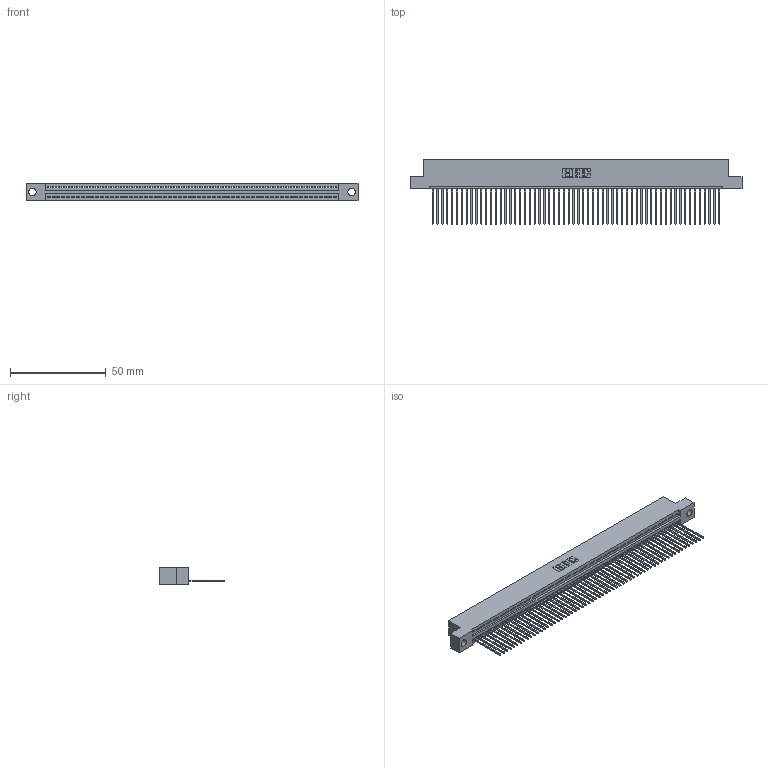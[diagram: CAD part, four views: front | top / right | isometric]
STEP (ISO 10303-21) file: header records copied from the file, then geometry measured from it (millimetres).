
FILE_DESCRIPTION (( 'STEP AP203' ), '1' );
FILE_NAME ('395-060-541-104.STEP', '2021-05-31T21:48:45', ( '' ), ( '' ), 'SwSTEP 2.0', 'SolidWorks 2020', '' );
FILE_SCHEMA (( 'CONFIG_CONTROL_DESIGN' ));
Length unit declared in the file: inch
Products named in the file (3): 345-292-001_345-293-141; 395-060-541-104; 345 Part_Flush Mounting Lugs - 0.156 Dia-TI
Assembly tree (61 placements, depth 2):
  395-060-541-104
    345 Part_Flush Mounting Lugs - 0.156 Dia-TI
    345-292-001_345-293-141  x60
Bounding box: 173.61 x 33.96 x 9.4 mm (x, y, z)
Volume: 16729.1 mm3; surface area: 23483.5 mm2
Topology: 61 solids, 61 shells, 3620 faces, 10937 edges, 7210 vertices
Faces by surface type: plane 2494, cylinder 1126
Entity records: 43171 total; most frequent: CARTESIAN_POINT 7486, ORIENTED_EDGE 7478, DIRECTION 6511, EDGE_CURVE 3739, VECTOR 3367, LINE 3367, VERTEX_POINT 2490, AXIS2_PLACEMENT_3D 1572
